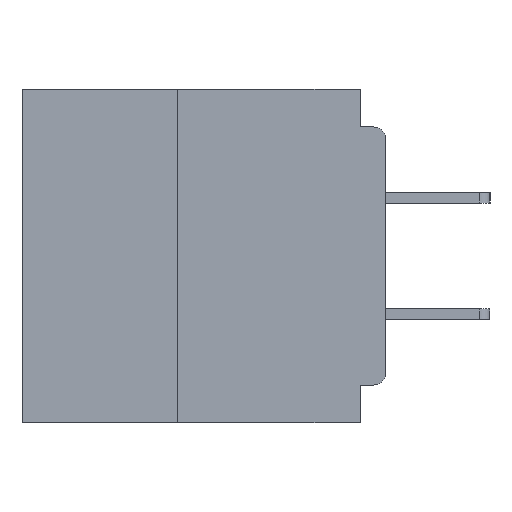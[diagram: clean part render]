
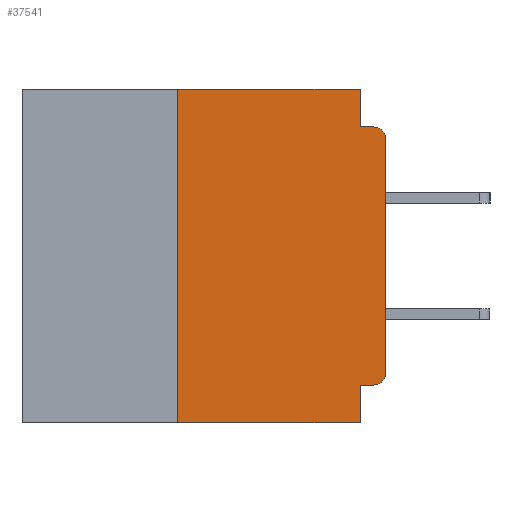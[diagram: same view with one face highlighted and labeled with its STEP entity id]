
A CAD part, left-side view. The second image highlights one B-rep face of the part: STEP entity #37541.
In plain terms, the highlighted planar face has unit normal (-1, 0, 0).
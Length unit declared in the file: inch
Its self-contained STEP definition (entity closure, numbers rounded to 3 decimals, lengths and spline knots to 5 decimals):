
#923 = VERTEX_POINT ( 'NONE', #57544 ) ;
#1557 = DIRECTION ( 'NONE',  ( 1., 0., 0. ) ) ;
#1824 = DIRECTION ( 'NONE',  ( 0., 0., -1. ) ) ;
#1836 = LINE ( 'NONE', #9527, #40181 ) ;
#2736 = DIRECTION ( 'NONE',  ( 0., -1., 0. ) ) ;
#3500 = VERTEX_POINT ( 'NONE', #56467 ) ;
#4580 = CARTESIAN_POINT ( 'NONE',  ( 0., 0.031, -0.4 ) ) ;
#8203 = VERTEX_POINT ( 'NONE', #58148 ) ;
#8495 = EDGE_CURVE ( 'NONE', #51720, #34768, #1836, .T. ) ;
#9109 = CARTESIAN_POINT ( 'NONE',  ( 0., 0.25, -0.4 ) ) ;
#9110 = CARTESIAN_POINT ( 'NONE',  ( 0., 0.031, -0.045 ) ) ;
#9527 = CARTESIAN_POINT ( 'NONE',  ( 0., 0.437, -0.4 ) ) ;
#10321 = CARTESIAN_POINT ( 'NONE',  ( 0., 0., -0.355 ) ) ;
#11392 = PLANE ( 'NONE',  #29612 ) ;
#11427 = DIRECTION ( 'NONE',  ( 0., 0., -1. ) ) ;
#12549 = CARTESIAN_POINT ( 'NONE',  ( 0., 0., -0.045 ) ) ;
#12552 = LINE ( 'NONE', #36392, #52512 ) ;
#12862 = EDGE_CURVE ( 'NONE', #51720, #56819, #50334, .T. ) ;
#13433 = LINE ( 'NONE', #16709, #51841 ) ;
#13722 = AXIS2_PLACEMENT_3D ( 'NONE', #17507, #52543, #22574 ) ;
#15088 = DIRECTION ( 'NONE',  ( -1., 0., 0. ) ) ;
#15363 = DIRECTION ( 'NONE',  ( 0., 1., 0. ) ) ;
#16129 = ORIENTED_EDGE ( 'NONE', *, *, #8495, .T. ) ;
#16382 = EDGE_CURVE ( 'NONE', #22932, #22431, #57656, .T. ) ;
#16709 = CARTESIAN_POINT ( 'NONE',  ( 0., 0.031, -0.4 ) ) ;
#17507 = CARTESIAN_POINT ( 'NONE',  ( 0., 0.015, -0.34 ) ) ;
#17688 = VECTOR ( 'NONE', #34025, 39.37008 ) ;
#18293 = ORIENTED_EDGE ( 'NONE', *, *, #24577, .T. ) ;
#18814 = CARTESIAN_POINT ( 'NONE',  ( 0., 0., -0.06 ) ) ;
#20245 = EDGE_CURVE ( 'NONE', #8203, #36642, #12552, .T. ) ;
#20900 = ORIENTED_EDGE ( 'NONE', *, *, #26673, .F. ) ;
#22431 = VERTEX_POINT ( 'NONE', #18814 ) ;
#22574 = DIRECTION ( 'NONE',  ( 0., 0., -1. ) ) ;
#22932 = VERTEX_POINT ( 'NONE', #47680 ) ;
#23688 = VECTOR ( 'NONE', #39028, 39.37008 ) ;
#24577 = EDGE_CURVE ( 'NONE', #3500, #22932, #62622, .T. ) ;
#24994 = DIRECTION ( 'NONE',  ( 0., -1., 0. ) ) ;
#26673 = EDGE_CURVE ( 'NONE', #36642, #923, #56806, .T. ) ;
#27000 = EDGE_CURVE ( 'NONE', #3500, #58329, #37278, .T. ) ;
#29612 = AXIS2_PLACEMENT_3D ( 'NONE', #31546, #1557, #36578 ) ;
#31530 = FACE_OUTER_BOUND ( 'NONE', #50122, .T. ) ;
#31546 = CARTESIAN_POINT ( 'NONE',  ( 0., 0.437, 0. ) ) ;
#34025 = DIRECTION ( 'NONE',  ( 0., 0., 1. ) ) ;
#34241 = CIRCLE ( 'NONE', #64334, 0.015 ) ;
#34506 = DIRECTION ( 'NONE',  ( 0., -1., 0. ) ) ;
#34614 = ORIENTED_EDGE ( 'NONE', *, *, #27000, .F. ) ;
#34768 = VERTEX_POINT ( 'NONE', #4580 ) ;
#35094 = CARTESIAN_POINT ( 'NONE',  ( 0., 0.437, 0. ) ) ;
#35408 = ORIENTED_EDGE ( 'NONE', *, *, #20245, .F. ) ;
#36392 = CARTESIAN_POINT ( 'NONE',  ( 0., 0.031, 0. ) ) ;
#36578 = DIRECTION ( 'NONE',  ( 0., 0., -1. ) ) ;
#36642 = VERTEX_POINT ( 'NONE', #9110 ) ;
#37221 = CARTESIAN_POINT ( 'NONE',  ( 0., 0.25, 0. ) ) ;
#37278 = LINE ( 'NONE', #10321, #62386 ) ;
#37541 = ADVANCED_FACE ( 'NONE', ( #31530 ), #11392, .F. ) ;
#38449 = LINE ( 'NONE', #35094, #50234 ) ;
#39018 = CARTESIAN_POINT ( 'NONE',  ( 0., 0., 0. ) ) ;
#39028 = DIRECTION ( 'NONE',  ( 0., 0., 1. ) ) ;
#40181 = VECTOR ( 'NONE', #34506, 39.37008 ) ;
#43477 = VECTOR ( 'NONE', #2736, 39.37008 ) ;
#45113 = CARTESIAN_POINT ( 'NONE',  ( 0., 0.015, -0.06 ) ) ;
#47680 = CARTESIAN_POINT ( 'NONE',  ( 0., 0., -0.34 ) ) ;
#48093 = EDGE_CURVE ( 'NONE', #58329, #34768, #13433, .T. ) ;
#50113 = DIRECTION ( 'NONE',  ( 0., 0., -1. ) ) ;
#50122 = EDGE_LOOP ( 'NONE', ( #54192, #61644, #20900, #35408, #50522, #62908, #16129, #62614, #34614, #18293 ) ) ;
#50234 = VECTOR ( 'NONE', #24994, 39.37008 ) ;
#50334 = LINE ( 'NONE', #54149, #23688 ) ;
#50522 = ORIENTED_EDGE ( 'NONE', *, *, #53642, .F. ) ;
#50976 = CARTESIAN_POINT ( 'NONE',  ( 0., 0.031, -0.355 ) ) ;
#51720 = VERTEX_POINT ( 'NONE', #9109 ) ;
#51841 = VECTOR ( 'NONE', #1824, 39.37008 ) ;
#52512 = VECTOR ( 'NONE', #11427, 39.37008 ) ;
#52543 = DIRECTION ( 'NONE',  ( -1., 0., 0. ) ) ;
#53642 = EDGE_CURVE ( 'NONE', #56819, #8203, #38449, .T. ) ;
#54149 = CARTESIAN_POINT ( 'NONE',  ( 0., 0.25, -0.4 ) ) ;
#54192 = ORIENTED_EDGE ( 'NONE', *, *, #16382, .T. ) ;
#56467 = CARTESIAN_POINT ( 'NONE',  ( 0., 0.015, -0.355 ) ) ;
#56806 = LINE ( 'NONE', #12549, #43477 ) ;
#56819 = VERTEX_POINT ( 'NONE', #37221 ) ;
#57544 = CARTESIAN_POINT ( 'NONE',  ( 0., 0.015, -0.045 ) ) ;
#57656 = LINE ( 'NONE', #39018, #17688 ) ;
#58148 = CARTESIAN_POINT ( 'NONE',  ( 0., 0.031, 0. ) ) ;
#58329 = VERTEX_POINT ( 'NONE', #50976 ) ;
#60140 = EDGE_CURVE ( 'NONE', #22431, #923, #34241, .T. ) ;
#61644 = ORIENTED_EDGE ( 'NONE', *, *, #60140, .T. ) ;
#62386 = VECTOR ( 'NONE', #15363, 39.37008 ) ;
#62614 = ORIENTED_EDGE ( 'NONE', *, *, #48093, .F. ) ;
#62622 = CIRCLE ( 'NONE', #13722, 0.015 ) ;
#62908 = ORIENTED_EDGE ( 'NONE', *, *, #12862, .F. ) ;
#64334 = AXIS2_PLACEMENT_3D ( 'NONE', #45113, #15088, #50113 ) ;
